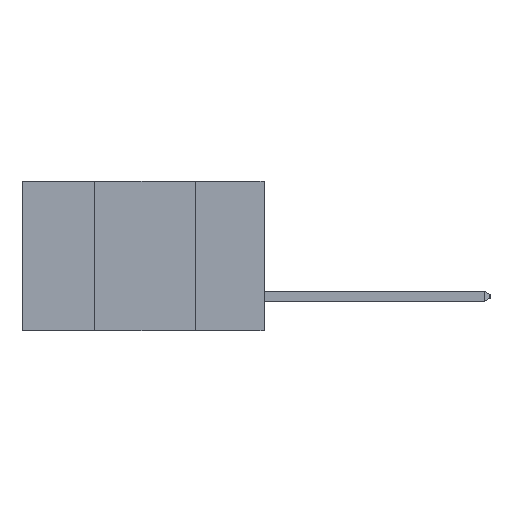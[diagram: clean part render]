
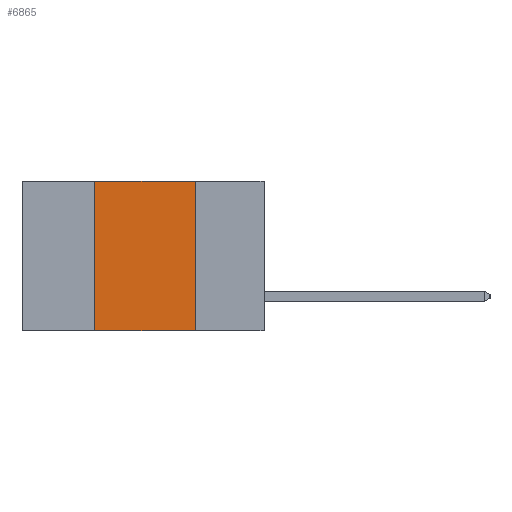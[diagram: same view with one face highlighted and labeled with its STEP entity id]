
A CAD part, left-side view. The second image highlights one B-rep face of the part: STEP entity #6865.
In plain terms, the highlighted planar face has unit normal (-1, 0, 0).
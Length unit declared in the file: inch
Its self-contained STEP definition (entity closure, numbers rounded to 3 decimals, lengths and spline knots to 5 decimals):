
#575 = VECTOR ( 'NONE', #3820, 39.37008 ) ;
#611 = LINE ( 'NONE', #8115, #2083 ) ;
#1108 = CARTESIAN_POINT ( 'NONE',  ( 0., 0.17, -0.37 ) ) ;
#1504 = CARTESIAN_POINT ( 'NONE',  ( 0., 0.17, -0.37 ) ) ;
#1544 = DIRECTION ( 'NONE',  ( 0., 0., 1. ) ) ;
#1623 = DIRECTION ( 'NONE',  ( 0., 0., -1. ) ) ;
#1692 = EDGE_CURVE ( 'NONE', #2613, #9035, #9581, .T. ) ;
#2032 = ORIENTED_EDGE ( 'NONE', *, *, #8672, .F. ) ;
#2083 = VECTOR ( 'NONE', #1544, 39.37008 ) ;
#2168 = ORIENTED_EDGE ( 'NONE', *, *, #1692, .F. ) ;
#2613 = VERTEX_POINT ( 'NONE', #6409 ) ;
#2925 = CARTESIAN_POINT ( 'NONE',  ( 0., 0.42, -0.37 ) ) ;
#2990 = EDGE_LOOP ( 'NONE', ( #2168, #4358, #2032, #9972 ) ) ;
#3020 = EDGE_CURVE ( 'NONE', #7313, #2613, #9293, .T. ) ;
#3102 = VECTOR ( 'NONE', #10595, 39.37008 ) ;
#3361 = VECTOR ( 'NONE', #1623, 39.37008 ) ;
#3681 = CARTESIAN_POINT ( 'NONE',  ( 0., 0.6, 0. ) ) ;
#3820 = DIRECTION ( 'NONE',  ( 0., -1., 0. ) ) ;
#4161 = AXIS2_PLACEMENT_3D ( 'NONE', #6912, #6507, #6335 ) ;
#4192 = VERTEX_POINT ( 'NONE', #2925 ) ;
#4358 = ORIENTED_EDGE ( 'NONE', *, *, #3020, .F. ) ;
#5302 = LINE ( 'NONE', #9005, #3102 ) ;
#6335 = DIRECTION ( 'NONE',  ( 0., 0., -1. ) ) ;
#6409 = CARTESIAN_POINT ( 'NONE',  ( 0., 0.17, 0. ) ) ;
#6507 = DIRECTION ( 'NONE',  ( 1., 0., 0. ) ) ;
#6577 = PLANE ( 'NONE',  #4161 ) ;
#6865 = ADVANCED_FACE ( 'NONE', ( #7771 ), #6577, .F. ) ;
#6912 = CARTESIAN_POINT ( 'NONE',  ( 0., 0.6, 0. ) ) ;
#7313 = VERTEX_POINT ( 'NONE', #8205 ) ;
#7771 = FACE_OUTER_BOUND ( 'NONE', #2990, .T. ) ;
#8115 = CARTESIAN_POINT ( 'NONE',  ( 0., 0.42, -0.37 ) ) ;
#8205 = CARTESIAN_POINT ( 'NONE',  ( 0., 0.42, 0. ) ) ;
#8672 = EDGE_CURVE ( 'NONE', #4192, #7313, #611, .T. ) ;
#9005 = CARTESIAN_POINT ( 'NONE',  ( 0., 0.6, -0.37 ) ) ;
#9035 = VERTEX_POINT ( 'NONE', #1108 ) ;
#9293 = LINE ( 'NONE', #3681, #575 ) ;
#9394 = EDGE_CURVE ( 'NONE', #4192, #9035, #5302, .T. ) ;
#9581 = LINE ( 'NONE', #1504, #3361 ) ;
#9972 = ORIENTED_EDGE ( 'NONE', *, *, #9394, .T. ) ;
#10595 = DIRECTION ( 'NONE',  ( 0., -1., 0. ) ) ;
